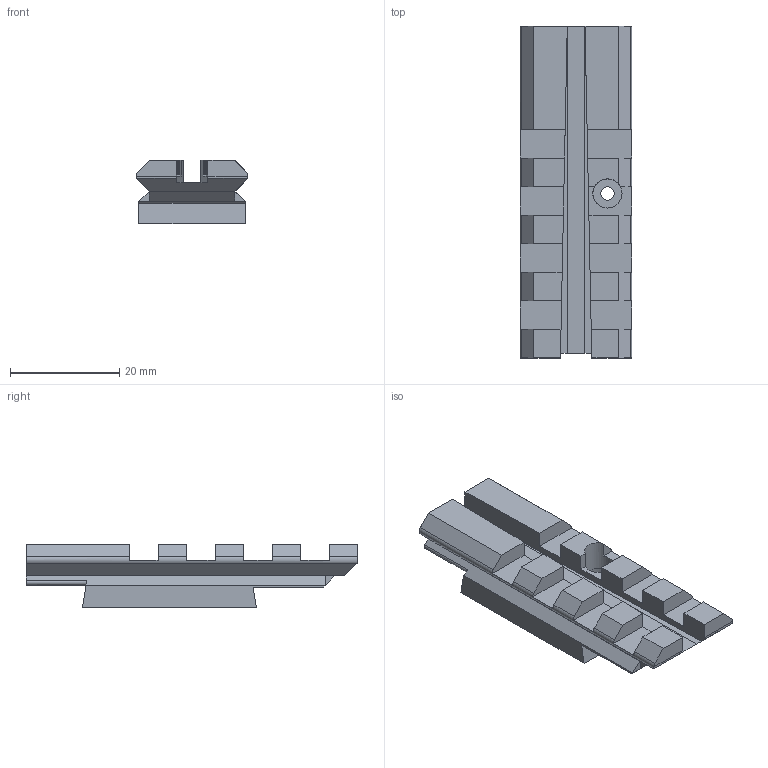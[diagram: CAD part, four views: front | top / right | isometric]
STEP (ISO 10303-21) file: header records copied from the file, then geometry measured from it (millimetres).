
FILE_DESCRIPTION(/* description */ (''),/* implementation_level */ '2;1');
FILE_NAME(/* name */ 'Pic Rail Adapter v7.step',/* time_stamp */ '2020-04-11T04:42:47-04:00',/* author */ (''),/* organization */ (''),/* preprocessor_version */ 'ST-DEVELOPER v18',/* originating_system */ 'Autodesk Translation Framework v8.12.0.6',/* authorisation */ '');
FILE_SCHEMA (('AUTOMOTIVE_DESIGN { 1 0 10303 214 3 1 1 }'));
Length unit declared in the file: millimetre
Products named in the file (1): Pic Rail Adapter
Bounding box: 20.45 x 60.81 x 11.69 mm (x, y, z)
Volume: 8552 mm3; surface area: 4755.6 mm2
Topology: 1 solids, 1 shells, 98 faces, 285 edges, 189 vertices
Faces by surface type: plane 91, cylinder 7
Full cylindrical faces by diameter (mm): 2.5 x1, 5.35 x2
Entity records: 3275 total; most frequent: CARTESIAN_POINT 575, ORIENTED_EDGE 574, DIRECTION 533, EDGE_CURVE 287, LINE 239, VECTOR 239, VERTEX_POINT 189, AXIS2_PLACEMENT_3D 147
